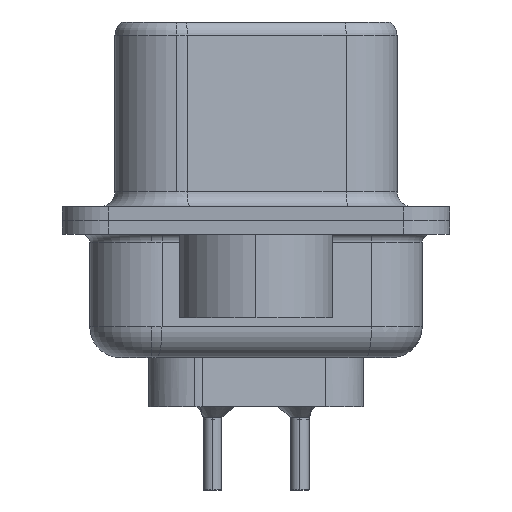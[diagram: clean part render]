
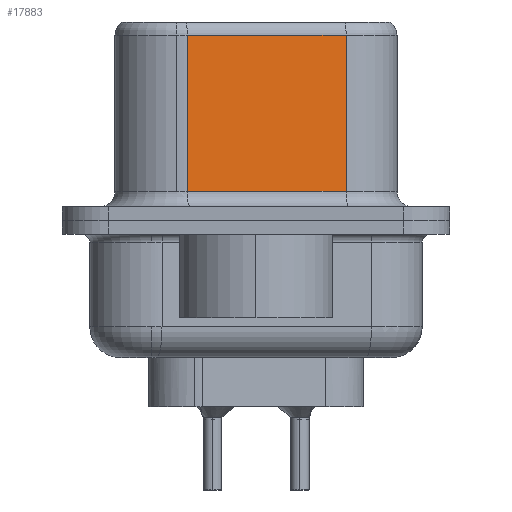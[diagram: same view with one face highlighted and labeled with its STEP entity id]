
A CAD part, left-side view. The second image highlights one B-rep face of the part: STEP entity #17883.
In plain terms, the highlighted planar face has unit normal (-0.985, -0.174, 0).
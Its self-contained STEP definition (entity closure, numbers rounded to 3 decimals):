
#1315 = DIRECTION ( 'NONE',  ( -0.174, 0.985, 0. ) ) ;
#1453 = AXIS2_PLACEMENT_3D ( 'NONE', #2171, #15770, #4085 ) ;
#1938 = VECTOR ( 'NONE', #1315, 1000. ) ;
#2171 = CARTESIAN_POINT ( 'NONE',  ( 4.58, -2.927, 6.52 ) ) ;
#2216 = CARTESIAN_POINT ( 'NONE',  ( 4.58, -2.927, 6.02 ) ) ;
#2667 = ORIENTED_EDGE ( 'NONE', *, *, #9136, .F. ) ;
#2816 = CARTESIAN_POINT ( 'NONE',  ( 4.58, -2.927, 0.95 ) ) ;
#2899 = DIRECTION ( 'NONE',  ( 0., 0., -1. ) ) ;
#3139 = VERTEX_POINT ( 'NONE', #24602 ) ;
#3781 = LINE ( 'NONE', #14816, #23918 ) ;
#4085 = DIRECTION ( 'NONE',  ( -0.174, 0.985, 0. ) ) ;
#4617 = DIRECTION ( 'NONE',  ( 0.174, -0.985, 0. ) ) ;
#5324 = VECTOR ( 'NONE', #4617, 1000. ) ;
#5419 = CARTESIAN_POINT ( 'NONE',  ( 3.67, 2.233, 0.95 ) ) ;
#5644 = FACE_OUTER_BOUND ( 'NONE', #12101, .T. ) ;
#7083 = LINE ( 'NONE', #7141, #1938 ) ;
#7141 = CARTESIAN_POINT ( 'NONE',  ( 4.58, -2.927, 6.02 ) ) ;
#9136 = EDGE_CURVE ( 'NONE', #21003, #3139, #3781, .T. ) ;
#11843 = ORIENTED_EDGE ( 'NONE', *, *, #12851, .T. ) ;
#12101 = EDGE_LOOP ( 'NONE', ( #2667, #11843, #14633, #17696 ) ) ;
#12304 = VERTEX_POINT ( 'NONE', #18992 ) ;
#12851 = EDGE_CURVE ( 'NONE', #21003, #12304, #7083, .T. ) ;
#14633 = ORIENTED_EDGE ( 'NONE', *, *, #22430, .T. ) ;
#14816 = CARTESIAN_POINT ( 'NONE',  ( 4.58, -2.927, 6.52 ) ) ;
#15053 = VERTEX_POINT ( 'NONE', #5419 ) ;
#15770 = DIRECTION ( 'NONE',  ( 0.985, 0.174, 0. ) ) ;
#17696 = ORIENTED_EDGE ( 'NONE', *, *, #22388, .T. ) ;
#17883 = ADVANCED_FACE ( 'NONE', ( #5644 ), #23527, .F. ) ;
#18448 = CARTESIAN_POINT ( 'NONE',  ( 3.67, 2.233, 6.52 ) ) ;
#18992 = CARTESIAN_POINT ( 'NONE',  ( 3.67, 2.233, 6.02 ) ) ;
#19047 = VECTOR ( 'NONE', #2899, 1000. ) ;
#21003 = VERTEX_POINT ( 'NONE', #2216 ) ;
#22146 = LINE ( 'NONE', #2816, #5324 ) ;
#22388 = EDGE_CURVE ( 'NONE', #15053, #3139, #22146, .T. ) ;
#22430 = EDGE_CURVE ( 'NONE', #12304, #15053, #24288, .T. ) ;
#22599 = DIRECTION ( 'NONE',  ( 0., 0., -1. ) ) ;
#23527 = PLANE ( 'NONE',  #1453 ) ;
#23918 = VECTOR ( 'NONE', #22599, 1000. ) ;
#24288 = LINE ( 'NONE', #18448, #19047 ) ;
#24602 = CARTESIAN_POINT ( 'NONE',  ( 4.58, -2.927, 0.95 ) ) ;
